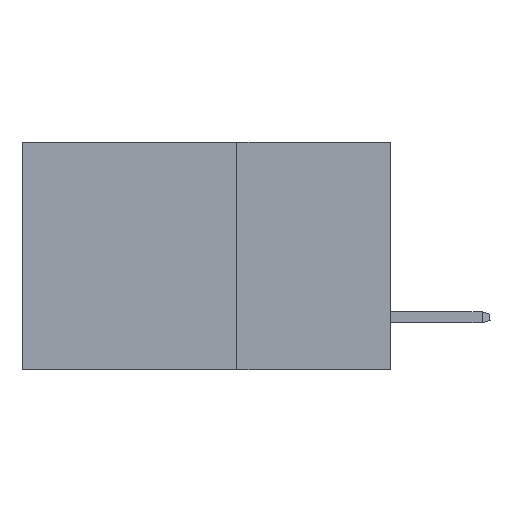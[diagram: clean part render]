
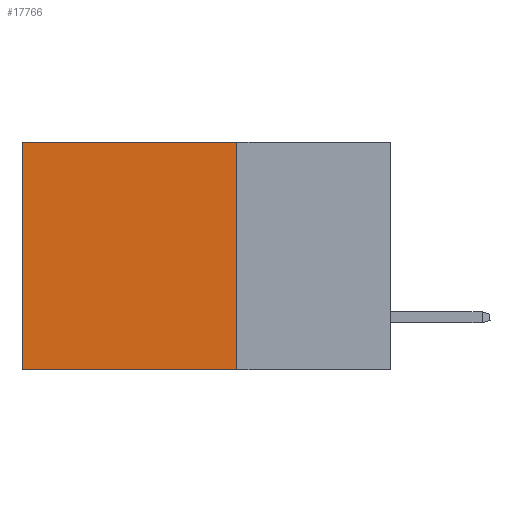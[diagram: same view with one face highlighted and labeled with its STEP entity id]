
A CAD part, left-side view. The second image highlights one B-rep face of the part: STEP entity #17766.
In plain terms, the highlighted planar face has unit normal (-1, 0, 0).
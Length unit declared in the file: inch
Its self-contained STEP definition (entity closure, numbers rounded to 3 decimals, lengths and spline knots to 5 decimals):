
#4433 = DIRECTION ( 'NONE',  ( 0., 1., 0. ) ) ;
#4566 = DIRECTION ( 'NONE',  ( 1., 0., 0. ) ) ;
#4706 = VECTOR ( 'NONE', #4433, 39.37008 ) ;
#5766 = DIRECTION ( 'NONE',  ( 0., 0., -1. ) ) ;
#9880 = CARTESIAN_POINT ( 'NONE',  ( 0.2875, 0.6, -0.37 ) ) ;
#10883 = CARTESIAN_POINT ( 'NONE',  ( 0.2875, 0.25, 0. ) ) ;
#14924 = CARTESIAN_POINT ( 'NONE',  ( 0.2875, 0.25, 0. ) ) ;
#15007 = VERTEX_POINT ( 'NONE', #29157 ) ;
#15497 = AXIS2_PLACEMENT_3D ( 'NONE', #10883, #4566, #23807 ) ;
#15820 = LINE ( 'NONE', #24090, #22357 ) ;
#17195 = EDGE_CURVE ( 'NONE', #22641, #15007, #31479, .T. ) ;
#17255 = VECTOR ( 'NONE', #5766, 39.37008 ) ;
#17766 = ADVANCED_FACE ( 'NONE', ( #28884 ), #20874, .F. ) ;
#17872 = EDGE_CURVE ( 'NONE', #15007, #32899, #15820, .T. ) ;
#20751 = EDGE_CURVE ( 'NONE', #22641, #29276, #33358, .T. ) ;
#20874 = PLANE ( 'NONE',  #15497 ) ;
#22357 = VECTOR ( 'NONE', #23534, 39.37008 ) ;
#22641 = VERTEX_POINT ( 'NONE', #14924 ) ;
#22819 = ORIENTED_EDGE ( 'NONE', *, *, #28354, .T. ) ;
#22925 = VECTOR ( 'NONE', #34820, 39.37008 ) ;
#23534 = DIRECTION ( 'NONE',  ( 0., 1., 0. ) ) ;
#23807 = DIRECTION ( 'NONE',  ( 0., 0., -1. ) ) ;
#24090 = CARTESIAN_POINT ( 'NONE',  ( 0.2875, 0.25, -0.37 ) ) ;
#24810 = LINE ( 'NONE', #40395, #17255 ) ;
#26293 = ORIENTED_EDGE ( 'NONE', *, *, #17872, .F. ) ;
#28354 = EDGE_CURVE ( 'NONE', #29276, #32899, #24810, .T. ) ;
#28481 = ORIENTED_EDGE ( 'NONE', *, *, #17195, .F. ) ;
#28788 = CARTESIAN_POINT ( 'NONE',  ( 0.2875, 0.25, 0. ) ) ;
#28884 = FACE_OUTER_BOUND ( 'NONE', #34677, .T. ) ;
#29157 = CARTESIAN_POINT ( 'NONE',  ( 0.2875, 0.25, -0.37 ) ) ;
#29276 = VERTEX_POINT ( 'NONE', #32933 ) ;
#31479 = LINE ( 'NONE', #28788, #22925 ) ;
#32898 = ORIENTED_EDGE ( 'NONE', *, *, #20751, .T. ) ;
#32899 = VERTEX_POINT ( 'NONE', #9880 ) ;
#32933 = CARTESIAN_POINT ( 'NONE',  ( 0.2875, 0.6, 0. ) ) ;
#33358 = LINE ( 'NONE', #36291, #4706 ) ;
#34677 = EDGE_LOOP ( 'NONE', ( #22819, #26293, #28481, #32898 ) ) ;
#34820 = DIRECTION ( 'NONE',  ( 0., 0., -1. ) ) ;
#36291 = CARTESIAN_POINT ( 'NONE',  ( 0.2875, 0.25, 0. ) ) ;
#40395 = CARTESIAN_POINT ( 'NONE',  ( 0.2875, 0.6, 0. ) ) ;
